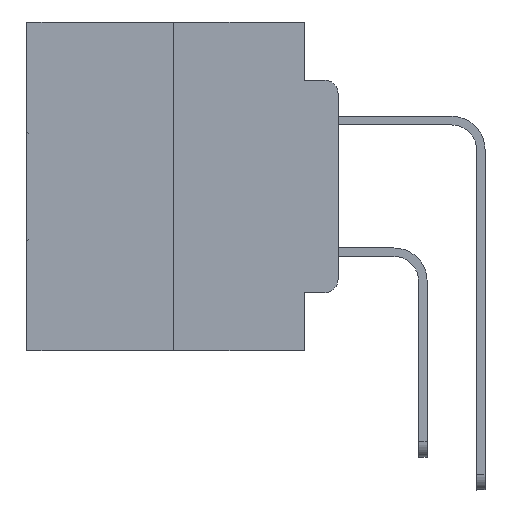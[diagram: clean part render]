
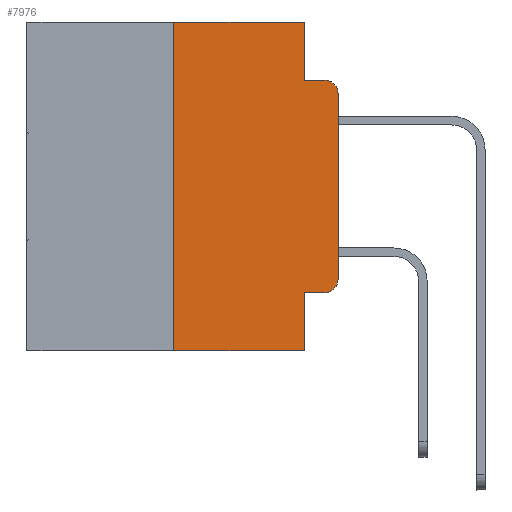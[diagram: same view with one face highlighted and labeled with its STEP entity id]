
A CAD part, left-side view. The second image highlights one B-rep face of the part: STEP entity #7976.
In plain terms, the highlighted planar face has unit normal (-1, 0, 0).
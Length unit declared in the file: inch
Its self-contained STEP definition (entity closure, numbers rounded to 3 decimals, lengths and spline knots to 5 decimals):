
#55 = CARTESIAN_POINT ( 'NONE',  ( 0., 0.051, 0. ) ) ;
#111 = VECTOR ( 'NONE', #9293, 39.37008 ) ;
#331 = VECTOR ( 'NONE', #7941, 39.37008 ) ;
#336 = DIRECTION ( 'NONE',  ( 0., 0., -1. ) ) ;
#558 = VERTEX_POINT ( 'NONE', #11797 ) ;
#1154 = VERTEX_POINT ( 'NONE', #23189 ) ;
#1407 = ORIENTED_EDGE ( 'NONE', *, *, #2189, .T. ) ;
#1809 = EDGE_CURVE ( 'NONE', #3027, #26598, #6464, .T. ) ;
#2189 = EDGE_CURVE ( 'NONE', #28541, #558, #16494, .T. ) ;
#3027 = VERTEX_POINT ( 'NONE', #7895 ) ;
#3767 = VERTEX_POINT ( 'NONE', #25111 ) ;
#3771 = EDGE_CURVE ( 'NONE', #3767, #28541, #20372, .T. ) ;
#4191 = VECTOR ( 'NONE', #7965, 39.37008 ) ;
#4282 = LINE ( 'NONE', #14423, #23349 ) ;
#5347 = ORIENTED_EDGE ( 'NONE', *, *, #19509, .F. ) ;
#5558 = CARTESIAN_POINT ( 'NONE',  ( 0., 0.02, -0.1085 ) ) ;
#6464 = CIRCLE ( 'NONE', #14834, 0.02 ) ;
#6557 = AXIS2_PLACEMENT_3D ( 'NONE', #7165, #19446, #24189 ) ;
#6789 = LINE ( 'NONE', #22316, #25725 ) ;
#7165 = CARTESIAN_POINT ( 'NONE',  ( 0., 0.02, -0.3915 ) ) ;
#7334 = VERTEX_POINT ( 'NONE', #55 ) ;
#7360 = DIRECTION ( 'NONE',  ( 0., 0., 1. ) ) ;
#7403 = ORIENTED_EDGE ( 'NONE', *, *, #15955, .T. ) ;
#7676 = CARTESIAN_POINT ( 'NONE',  ( 0., 0., 0. ) ) ;
#7895 = CARTESIAN_POINT ( 'NONE',  ( 0., 0., -0.1085 ) ) ;
#7898 = DIRECTION ( 'NONE',  ( 1., 0., 0. ) ) ;
#7941 = DIRECTION ( 'NONE',  ( 0., -1., 0. ) ) ;
#7965 = DIRECTION ( 'NONE',  ( 0., -1., 0. ) ) ;
#7976 = ADVANCED_FACE ( 'NONE', ( #15276 ), #12799, .F. ) ;
#8254 = VERTEX_POINT ( 'NONE', #29767 ) ;
#8915 = CARTESIAN_POINT ( 'NONE',  ( 0., 0.02, -0.4115 ) ) ;
#9293 = DIRECTION ( 'NONE',  ( 0., 0., -1. ) ) ;
#9957 = LINE ( 'NONE', #31696, #111 ) ;
#11699 = CARTESIAN_POINT ( 'NONE',  ( 0., 0.051, -0.0885 ) ) ;
#11797 = CARTESIAN_POINT ( 'NONE',  ( 0., 0., -0.3915 ) ) ;
#12451 = ORIENTED_EDGE ( 'NONE', *, *, #21784, .F. ) ;
#12498 = AXIS2_PLACEMENT_3D ( 'NONE', #22775, #7898, #336 ) ;
#12651 = VECTOR ( 'NONE', #27055, 39.37008 ) ;
#12799 = PLANE ( 'NONE',  #12498 ) ;
#13174 = VERTEX_POINT ( 'NONE', #19358 ) ;
#13713 = ORIENTED_EDGE ( 'NONE', *, *, #19640, .F. ) ;
#14221 = VECTOR ( 'NONE', #7360, 39.37008 ) ;
#14320 = DIRECTION ( 'NONE',  ( 0., 0., 1. ) ) ;
#14423 = CARTESIAN_POINT ( 'NONE',  ( 0., 0.051, 0. ) ) ;
#14713 = CARTESIAN_POINT ( 'NONE',  ( 0., 0.02, -0.0885 ) ) ;
#14834 = AXIS2_PLACEMENT_3D ( 'NONE', #5558, #30076, #22731 ) ;
#15276 = FACE_OUTER_BOUND ( 'NONE', #19721, .T. ) ;
#15955 = EDGE_CURVE ( 'NONE', #13174, #8254, #17569, .T. ) ;
#16494 = CIRCLE ( 'NONE', #6557, 0.02 ) ;
#16619 = LINE ( 'NONE', #17107, #12651 ) ;
#17107 = CARTESIAN_POINT ( 'NONE',  ( 0., 0.473, 0. ) ) ;
#17569 = LINE ( 'NONE', #27683, #30749 ) ;
#17617 = LINE ( 'NONE', #18103, #4191 ) ;
#17785 = EDGE_CURVE ( 'NONE', #18185, #26598, #17617, .T. ) ;
#18103 = CARTESIAN_POINT ( 'NONE',  ( 0., 0.051, -0.0885 ) ) ;
#18185 = VERTEX_POINT ( 'NONE', #11699 ) ;
#19272 = EDGE_CURVE ( 'NONE', #558, #3027, #29588, .T. ) ;
#19358 = CARTESIAN_POINT ( 'NONE',  ( 0., 0.25, -0.5 ) ) ;
#19446 = DIRECTION ( 'NONE',  ( -1., 0., 0. ) ) ;
#19509 = EDGE_CURVE ( 'NONE', #1154, #7334, #16619, .T. ) ;
#19640 = EDGE_CURVE ( 'NONE', #13174, #1154, #6789, .T. ) ;
#19721 = EDGE_LOOP ( 'NONE', ( #25410, #28300, #27824, #12451, #5347, #13713, #7403, #30910, #21570, #1407 ) ) ;
#20372 = LINE ( 'NONE', #20533, #331 ) ;
#20533 = CARTESIAN_POINT ( 'NONE',  ( 0., 0.051, -0.4115 ) ) ;
#21570 = ORIENTED_EDGE ( 'NONE', *, *, #3771, .T. ) ;
#21784 = EDGE_CURVE ( 'NONE', #7334, #18185, #9957, .T. ) ;
#21945 = DIRECTION ( 'NONE',  ( 0., 0., -1. ) ) ;
#22316 = CARTESIAN_POINT ( 'NONE',  ( 0., 0.25, 0. ) ) ;
#22731 = DIRECTION ( 'NONE',  ( 0., 0., -1. ) ) ;
#22775 = CARTESIAN_POINT ( 'NONE',  ( 0., 0.473, 0. ) ) ;
#23189 = CARTESIAN_POINT ( 'NONE',  ( 0., 0.25, 0. ) ) ;
#23349 = VECTOR ( 'NONE', #21945, 39.37008 ) ;
#24189 = DIRECTION ( 'NONE',  ( 0., 0., -1. ) ) ;
#25111 = CARTESIAN_POINT ( 'NONE',  ( 0., 0.051, -0.4115 ) ) ;
#25410 = ORIENTED_EDGE ( 'NONE', *, *, #19272, .T. ) ;
#25708 = EDGE_CURVE ( 'NONE', #3767, #8254, #4282, .T. ) ;
#25725 = VECTOR ( 'NONE', #14320, 39.37008 ) ;
#26598 = VERTEX_POINT ( 'NONE', #14713 ) ;
#27055 = DIRECTION ( 'NONE',  ( 0., -1., 0. ) ) ;
#27683 = CARTESIAN_POINT ( 'NONE',  ( 0., 0.473, -0.5 ) ) ;
#27824 = ORIENTED_EDGE ( 'NONE', *, *, #17785, .F. ) ;
#28300 = ORIENTED_EDGE ( 'NONE', *, *, #1809, .T. ) ;
#28541 = VERTEX_POINT ( 'NONE', #8915 ) ;
#29588 = LINE ( 'NONE', #7676, #14221 ) ;
#29767 = CARTESIAN_POINT ( 'NONE',  ( 0., 0.051, -0.5 ) ) ;
#30076 = DIRECTION ( 'NONE',  ( -1., 0., 0. ) ) ;
#30629 = DIRECTION ( 'NONE',  ( 0., -1., 0. ) ) ;
#30749 = VECTOR ( 'NONE', #30629, 39.37008 ) ;
#30910 = ORIENTED_EDGE ( 'NONE', *, *, #25708, .F. ) ;
#31696 = CARTESIAN_POINT ( 'NONE',  ( 0., 0.051, 0. ) ) ;
